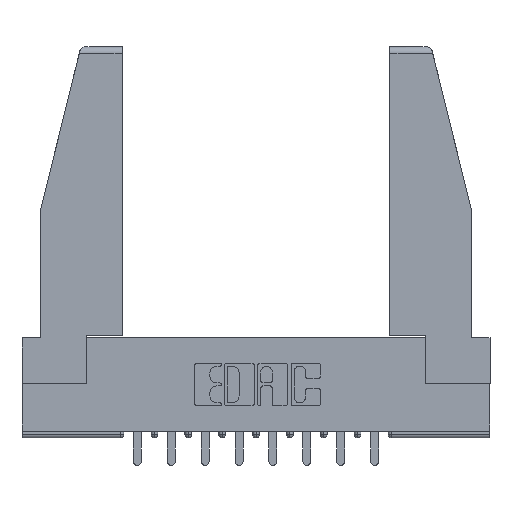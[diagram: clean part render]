
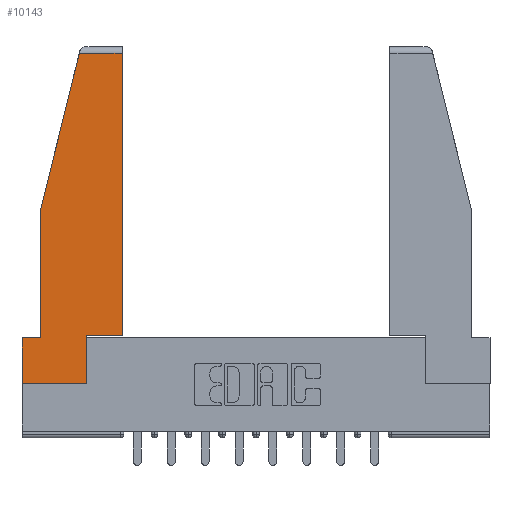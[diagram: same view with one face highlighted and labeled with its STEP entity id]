
A CAD part, top view. The second image highlights one B-rep face of the part: STEP entity #10143.
In plain terms, the highlighted planar face has unit normal (0, 0, 1).
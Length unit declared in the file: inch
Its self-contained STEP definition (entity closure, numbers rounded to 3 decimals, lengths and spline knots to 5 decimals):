
#209 = ORIENTED_EDGE ( 'NONE', *, *, #10562, .T. ) ;
#1220 = LINE ( 'NONE', #3166, #6740 ) ;
#1327 = CARTESIAN_POINT ( 'NONE',  ( 0.461, 1.52, 0. ) ) ;
#1514 = LINE ( 'NONE', #7811, #12383 ) ;
#1690 = VECTOR ( 'NONE', #3387, 39.37008 ) ;
#1828 = DIRECTION ( 'NONE',  ( -0.239, -0.971, 0. ) ) ;
#1840 = ORIENTED_EDGE ( 'NONE', *, *, #9375, .T. ) ;
#1912 = CARTESIAN_POINT ( 'NONE',  ( 0.461, 0.223, 0. ) ) ;
#1931 = LINE ( 'NONE', #6494, #11209 ) ;
#2212 = VERTEX_POINT ( 'NONE', #1327 ) ;
#2246 = FACE_OUTER_BOUND ( 'NONE', #3321, .T. ) ;
#2388 = CARTESIAN_POINT ( 'NONE',  ( 0.461, 0.223, 0. ) ) ;
#2389 = LINE ( 'NONE', #6943, #7970 ) ;
#2491 = DIRECTION ( 'NONE',  ( 0., -1., 0. ) ) ;
#2529 = VERTEX_POINT ( 'NONE', #2538 ) ;
#2538 = CARTESIAN_POINT ( 'NONE',  ( 0., 0.21, 0. ) ) ;
#2612 = VECTOR ( 'NONE', #1828, 39.37008 ) ;
#2790 = EDGE_CURVE ( 'NONE', #3954, #7055, #13131, .T. ) ;
#3166 = CARTESIAN_POINT ( 'NONE',  ( 0., 1.52, 0. ) ) ;
#3224 = DIRECTION ( 'NONE',  ( 1., 0., 0. ) ) ;
#3234 = LINE ( 'NONE', #6717, #1690 ) ;
#3252 = CARTESIAN_POINT ( 'NONE',  ( 0.086, 0.8, 0. ) ) ;
#3321 = EDGE_LOOP ( 'NONE', ( #12717, #7582, #13356, #7849, #209, #4873, #1840, #10339, #4683 ) ) ;
#3387 = DIRECTION ( 'NONE',  ( -1., 0., 0. ) ) ;
#3654 = LINE ( 'NONE', #5900, #10039 ) ;
#3954 = VERTEX_POINT ( 'NONE', #14138 ) ;
#4410 = DIRECTION ( 'NONE',  ( 1., 0., 0. ) ) ;
#4683 = ORIENTED_EDGE ( 'NONE', *, *, #2790, .T. ) ;
#4712 = DIRECTION ( 'NONE',  ( 1., 0., 0. ) ) ;
#4873 = ORIENTED_EDGE ( 'NONE', *, *, #8530, .T. ) ;
#5153 = CARTESIAN_POINT ( 'NONE',  ( 0.086, 0.21, 0. ) ) ;
#5252 = DIRECTION ( 'NONE',  ( 0., 1., 0. ) ) ;
#5283 = VERTEX_POINT ( 'NONE', #12537 ) ;
#5790 = VERTEX_POINT ( 'NONE', #12785 ) ;
#5900 = CARTESIAN_POINT ( 'NONE',  ( 0.086, 0.8, 0. ) ) ;
#5967 = EDGE_CURVE ( 'NONE', #2212, #7109, #1220, .T. ) ;
#6176 = EDGE_CURVE ( 'NONE', #7055, #2212, #11819, .T. ) ;
#6266 = VECTOR ( 'NONE', #5252, 39.37008 ) ;
#6494 = CARTESIAN_POINT ( 'NONE',  ( 0., 0.21, 0. ) ) ;
#6717 = CARTESIAN_POINT ( 'NONE',  ( 0., 0.21, 0. ) ) ;
#6740 = VECTOR ( 'NONE', #14227, 39.37008 ) ;
#6808 = DIRECTION ( 'NONE',  ( 0., 0., 1. ) ) ;
#6943 = CARTESIAN_POINT ( 'NONE',  ( 0., 0., 0. ) ) ;
#7055 = VERTEX_POINT ( 'NONE', #2388 ) ;
#7109 = VERTEX_POINT ( 'NONE', #11229 ) ;
#7319 = LINE ( 'NONE', #11741, #2612 ) ;
#7582 = ORIENTED_EDGE ( 'NONE', *, *, #5967, .T. ) ;
#7811 = CARTESIAN_POINT ( 'NONE',  ( 0.297, 0., 0. ) ) ;
#7849 = ORIENTED_EDGE ( 'NONE', *, *, #9155, .T. ) ;
#7922 = CARTESIAN_POINT ( 'NONE',  ( 0.297, 0.223, 0. ) ) ;
#7970 = VECTOR ( 'NONE', #4712, 39.37008 ) ;
#8530 = EDGE_CURVE ( 'NONE', #2529, #5790, #1931, .T. ) ;
#9155 = EDGE_CURVE ( 'NONE', #9301, #9265, #3654, .T. ) ;
#9265 = VERTEX_POINT ( 'NONE', #5153 ) ;
#9301 = VERTEX_POINT ( 'NONE', #3252 ) ;
#9375 = EDGE_CURVE ( 'NONE', #5790, #5283, #2389, .T. ) ;
#10039 = VECTOR ( 'NONE', #2491, 39.37008 ) ;
#10143 = ADVANCED_FACE ( 'NONE', ( #2246 ), #11154, .T. ) ;
#10339 = ORIENTED_EDGE ( 'NONE', *, *, #13370, .T. ) ;
#10562 = EDGE_CURVE ( 'NONE', #9265, #2529, #3234, .T. ) ;
#10840 = DIRECTION ( 'NONE',  ( 0., -1., 0. ) ) ;
#11154 = PLANE ( 'NONE',  #12566 ) ;
#11209 = VECTOR ( 'NONE', #10840, 39.37008 ) ;
#11229 = CARTESIAN_POINT ( 'NONE',  ( 0.2636, 1.52, 0. ) ) ;
#11331 = EDGE_CURVE ( 'NONE', #7109, #9301, #7319, .T. ) ;
#11741 = CARTESIAN_POINT ( 'NONE',  ( 0.271, 1.55, 0. ) ) ;
#11819 = LINE ( 'NONE', #1912, #6266 ) ;
#12232 = DIRECTION ( 'NONE',  ( 0., 1., 0. ) ) ;
#12383 = VECTOR ( 'NONE', #12232, 39.37008 ) ;
#12537 = CARTESIAN_POINT ( 'NONE',  ( 0.297, 0., 0. ) ) ;
#12566 = AXIS2_PLACEMENT_3D ( 'NONE', #13379, #6808, #4410 ) ;
#12717 = ORIENTED_EDGE ( 'NONE', *, *, #6176, .T. ) ;
#12785 = CARTESIAN_POINT ( 'NONE',  ( 0., 0., 0. ) ) ;
#13131 = LINE ( 'NONE', #7922, #14065 ) ;
#13356 = ORIENTED_EDGE ( 'NONE', *, *, #11331, .T. ) ;
#13370 = EDGE_CURVE ( 'NONE', #5283, #3954, #1514, .T. ) ;
#13379 = CARTESIAN_POINT ( 'NONE',  ( 0., 0., 0. ) ) ;
#14065 = VECTOR ( 'NONE', #3224, 39.37008 ) ;
#14138 = CARTESIAN_POINT ( 'NONE',  ( 0.297, 0.223, 0. ) ) ;
#14227 = DIRECTION ( 'NONE',  ( -1., 0., 0. ) ) ;
